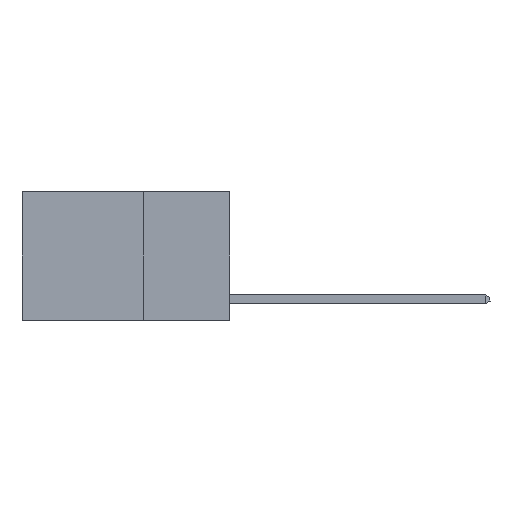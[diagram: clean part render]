
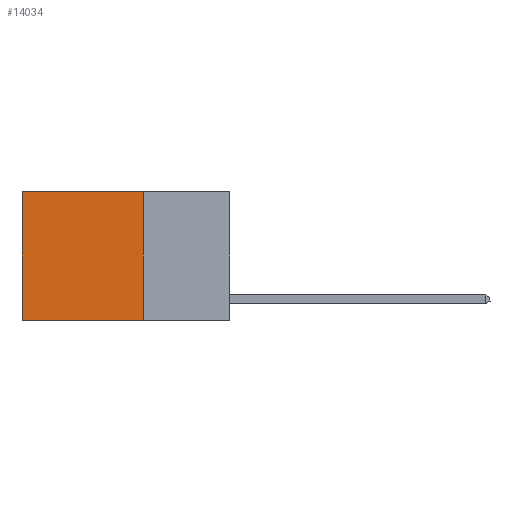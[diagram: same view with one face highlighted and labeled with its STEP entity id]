
A CAD part, left-side view. The second image highlights one B-rep face of the part: STEP entity #14034.
In plain terms, the highlighted planar face has unit normal (-1, 0, 0).
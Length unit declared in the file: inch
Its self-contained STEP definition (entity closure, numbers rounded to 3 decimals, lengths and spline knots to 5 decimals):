
#1052 = LINE ( 'NONE', #8962, #14022 ) ;
#1134 = VERTEX_POINT ( 'NONE', #14262 ) ;
#1603 = CARTESIAN_POINT ( 'NONE',  ( 0.2625, 0.25, 0. ) ) ;
#3521 = ORIENTED_EDGE ( 'NONE', *, *, #10515, .T. ) ;
#3707 = CARTESIAN_POINT ( 'NONE',  ( 0.2625, 0.25, -0.37 ) ) ;
#3709 = CARTESIAN_POINT ( 'NONE',  ( 0.2625, 0.6, -0.37 ) ) ;
#3877 = VERTEX_POINT ( 'NONE', #3707 ) ;
#4370 = DIRECTION ( 'NONE',  ( 0., 1., 0. ) ) ;
#4509 = VECTOR ( 'NONE', #6055, 39.37008 ) ;
#4537 = ORIENTED_EDGE ( 'NONE', *, *, #9651, .F. ) ;
#4857 = AXIS2_PLACEMENT_3D ( 'NONE', #1603, #11427, #12659 ) ;
#4967 = LINE ( 'NONE', #13721, #4509 ) ;
#6055 = DIRECTION ( 'NONE',  ( 0., 1., 0. ) ) ;
#6433 = VERTEX_POINT ( 'NONE', #3709 ) ;
#7440 = EDGE_CURVE ( 'NONE', #9677, #6433, #10680, .T. ) ;
#7449 = CARTESIAN_POINT ( 'NONE',  ( 0.2625, 0.25, 0. ) ) ;
#7519 = LINE ( 'NONE', #7449, #7822 ) ;
#7712 = CARTESIAN_POINT ( 'NONE',  ( 0.2625, 0.6, 0. ) ) ;
#7822 = VECTOR ( 'NONE', #11986, 39.37008 ) ;
#8259 = EDGE_CURVE ( 'NONE', #1134, #3877, #7519, .T. ) ;
#8962 = CARTESIAN_POINT ( 'NONE',  ( 0.2625, 0.25, -0.37 ) ) ;
#9075 = PLANE ( 'NONE',  #4857 ) ;
#9176 = ORIENTED_EDGE ( 'NONE', *, *, #8259, .F. ) ;
#9651 = EDGE_CURVE ( 'NONE', #3877, #6433, #1052, .T. ) ;
#9677 = VERTEX_POINT ( 'NONE', #7712 ) ;
#10488 = ORIENTED_EDGE ( 'NONE', *, *, #7440, .T. ) ;
#10515 = EDGE_CURVE ( 'NONE', #1134, #9677, #4967, .T. ) ;
#10531 = CARTESIAN_POINT ( 'NONE',  ( 0.2625, 0.6, 0. ) ) ;
#10680 = LINE ( 'NONE', #10531, #11780 ) ;
#11427 = DIRECTION ( 'NONE',  ( 1., 0., 0. ) ) ;
#11449 = EDGE_LOOP ( 'NONE', ( #10488, #4537, #9176, #3521 ) ) ;
#11501 = FACE_OUTER_BOUND ( 'NONE', #11449, .T. ) ;
#11780 = VECTOR ( 'NONE', #13798, 39.37008 ) ;
#11986 = DIRECTION ( 'NONE',  ( 0., 0., -1. ) ) ;
#12659 = DIRECTION ( 'NONE',  ( 0., 0., -1. ) ) ;
#13721 = CARTESIAN_POINT ( 'NONE',  ( 0.2625, 0.25, 0. ) ) ;
#13798 = DIRECTION ( 'NONE',  ( 0., 0., -1. ) ) ;
#14022 = VECTOR ( 'NONE', #4370, 39.37008 ) ;
#14034 = ADVANCED_FACE ( 'NONE', ( #11501 ), #9075, .F. ) ;
#14262 = CARTESIAN_POINT ( 'NONE',  ( 0.2625, 0.25, 0. ) ) ;
